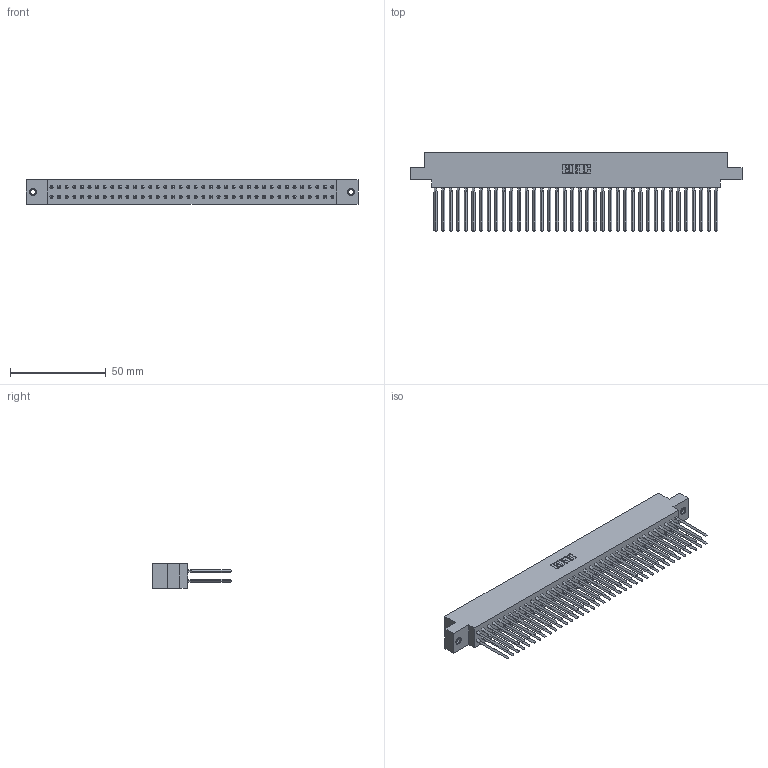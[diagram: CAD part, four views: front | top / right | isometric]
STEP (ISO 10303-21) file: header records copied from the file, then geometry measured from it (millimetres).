
FILE_DESCRIPTION (( 'STEP AP203' ), '1' );
FILE_NAME ('317-076-543-807.STEP', '2020-02-28T08:34:09', ( '' ), ( '' ), 'SwSTEP 2.0', 'SolidWorks 2016', '' );
FILE_SCHEMA (( 'CONFIG_CONTROL_DESIGN' ));
Length unit declared in the file: inch
Products named in the file (4): 345-250-001_345-250-005-103; 317-076-543-807; 317 Part_.156 Dia - TI; 317-290-001_543
Assembly tree (79 placements, depth 2):
  317-076-543-807
    317 Part_.156 Dia - TI
    317-290-001_543  x76
    345-250-001_345-250-005-103  x2
Bounding box: 173.28 x 41.15 x 12.7 mm (x, y, z)
Volume: 29311 mm3; surface area: 44345.8 mm2
Topology: 79 solids, 79 shells, 6926 faces, 19183 edges, 12350 vertices
Faces by surface type: plane 5638, cylinder 968, bspline 304, cone 12, torus 4
Entity records: 56673 total; most frequent: CARTESIAN_POINT 10274, ORIENTED_EDGE 9766, DIRECTION 8187, EDGE_CURVE 4883, LINE 4607, VECTOR 4607, VERTEX_POINT 3245, AXIS2_PLACEMENT_3D 1790
